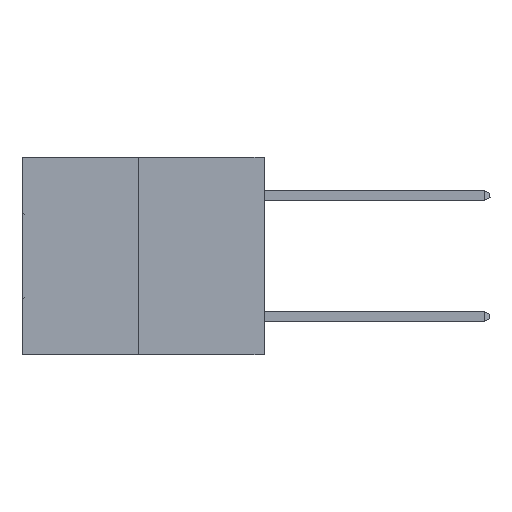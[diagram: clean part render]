
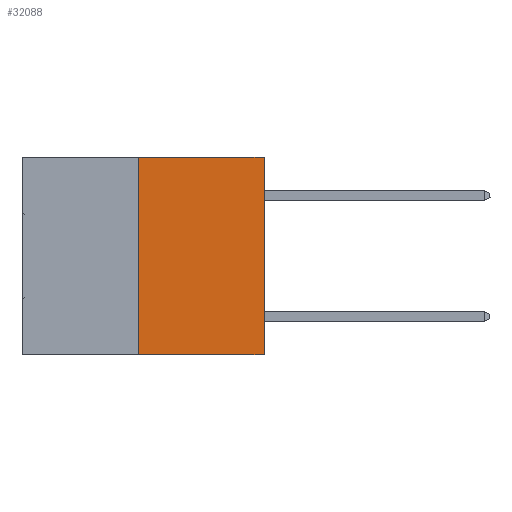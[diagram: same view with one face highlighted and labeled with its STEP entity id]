
A CAD part, left-side view. The second image highlights one B-rep face of the part: STEP entity #32088.
In plain terms, the highlighted planar face has unit normal (-1, 0, 0).
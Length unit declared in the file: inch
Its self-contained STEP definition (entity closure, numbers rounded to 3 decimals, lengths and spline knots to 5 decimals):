
#502 = VERTEX_POINT ( 'NONE', #1604 ) ;
#1604 = CARTESIAN_POINT ( 'NONE',  ( 0., 0.312, 0. ) ) ;
#2269 = CARTESIAN_POINT ( 'NONE',  ( 0., 0.312, -0.49 ) ) ;
#3796 = DIRECTION ( 'NONE',  ( 0., 0., -1. ) ) ;
#4724 = LINE ( 'NONE', #2269, #33724 ) ;
#6278 = VECTOR ( 'NONE', #28980, 39.37008 ) ;
#7179 = CARTESIAN_POINT ( 'NONE',  ( 0., 0., 0. ) ) ;
#7340 = EDGE_CURVE ( 'NONE', #13958, #22467, #13267, .T. ) ;
#8861 = CARTESIAN_POINT ( 'NONE',  ( 0., 0., -0.49 ) ) ;
#9639 = PLANE ( 'NONE',  #33211 ) ;
#11889 = EDGE_CURVE ( 'NONE', #502, #22467, #29809, .T. ) ;
#13267 = LINE ( 'NONE', #20038, #6278 ) ;
#13958 = VERTEX_POINT ( 'NONE', #8861 ) ;
#14403 = LINE ( 'NONE', #28516, #29062 ) ;
#14983 = FACE_OUTER_BOUND ( 'NONE', #26276, .T. ) ;
#20038 = CARTESIAN_POINT ( 'NONE',  ( 0., 0., 0. ) ) ;
#22467 = VERTEX_POINT ( 'NONE', #7179 ) ;
#24335 = DIRECTION ( 'NONE',  ( 0., -1., 0. ) ) ;
#24395 = EDGE_CURVE ( 'NONE', #28903, #13958, #14403, .T. ) ;
#24424 = EDGE_CURVE ( 'NONE', #28903, #502, #4724, .T. ) ;
#24582 = CARTESIAN_POINT ( 'NONE',  ( 0., 0.6, 0. ) ) ;
#25147 = ORIENTED_EDGE ( 'NONE', *, *, #7340, .T. ) ;
#25189 = ORIENTED_EDGE ( 'NONE', *, *, #24424, .F. ) ;
#25681 = DIRECTION ( 'NONE',  ( 0., -1., 0. ) ) ;
#26222 = ORIENTED_EDGE ( 'NONE', *, *, #11889, .F. ) ;
#26276 = EDGE_LOOP ( 'NONE', ( #25189, #33319, #25147, #26222 ) ) ;
#27035 = VECTOR ( 'NONE', #24335, 39.37008 ) ;
#28516 = CARTESIAN_POINT ( 'NONE',  ( 0., 0.6, -0.49 ) ) ;
#28756 = DIRECTION ( 'NONE',  ( 0., 0., 1. ) ) ;
#28903 = VERTEX_POINT ( 'NONE', #31556 ) ;
#28980 = DIRECTION ( 'NONE',  ( 0., 0., 1. ) ) ;
#29062 = VECTOR ( 'NONE', #25681, 39.37008 ) ;
#29809 = LINE ( 'NONE', #24582, #27035 ) ;
#30428 = DIRECTION ( 'NONE',  ( 1., 0., 0. ) ) ;
#31556 = CARTESIAN_POINT ( 'NONE',  ( 0., 0.312, -0.49 ) ) ;
#32088 = ADVANCED_FACE ( 'NONE', ( #14983 ), #9639, .F. ) ;
#33001 = CARTESIAN_POINT ( 'NONE',  ( 0., 0.6, 0. ) ) ;
#33211 = AXIS2_PLACEMENT_3D ( 'NONE', #33001, #30428, #3796 ) ;
#33319 = ORIENTED_EDGE ( 'NONE', *, *, #24395, .T. ) ;
#33724 = VECTOR ( 'NONE', #28756, 39.37008 ) ;
